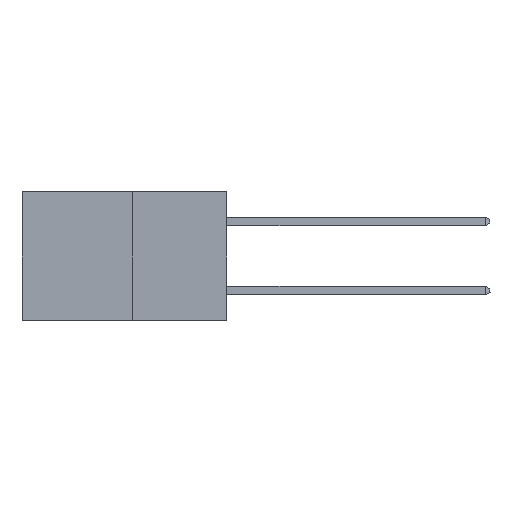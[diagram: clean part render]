
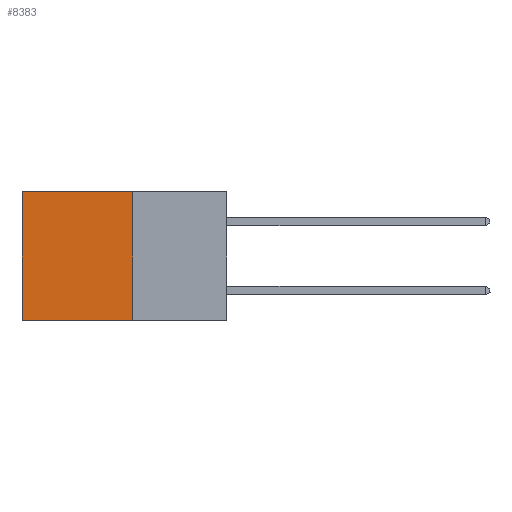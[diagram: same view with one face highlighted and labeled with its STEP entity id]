
A CAD part, left-side view. The second image highlights one B-rep face of the part: STEP entity #8383.
In plain terms, the highlighted planar face has unit normal (-1, 0, 0).
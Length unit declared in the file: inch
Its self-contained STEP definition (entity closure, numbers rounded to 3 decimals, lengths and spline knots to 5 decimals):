
#477 = ORIENTED_EDGE ( 'NONE', *, *, #12826, .F. ) ;
#1267 = VECTOR ( 'NONE', #27834, 39.37008 ) ;
#1766 = DIRECTION ( 'NONE',  ( 0., 0., -1. ) ) ;
#3061 = EDGE_CURVE ( 'NONE', #23658, #22537, #20502, .T. ) ;
#3997 = CARTESIAN_POINT ( 'NONE',  ( 0.277, 0.59, -0.37 ) ) ;
#6539 = LINE ( 'NONE', #20840, #18861 ) ;
#6622 = DIRECTION ( 'NONE',  ( 0., 0., -1. ) ) ;
#6968 = DIRECTION ( 'NONE',  ( 0., 0., -1. ) ) ;
#8383 = ADVANCED_FACE ( 'NONE', ( #29174 ), #13370, .F. ) ;
#8537 = EDGE_CURVE ( 'NONE', #22537, #20049, #6539, .T. ) ;
#9358 = CARTESIAN_POINT ( 'NONE',  ( 0.277, 0.27, -0.37 ) ) ;
#9962 = CARTESIAN_POINT ( 'NONE',  ( 0.277, 0.27, 0. ) ) ;
#10713 = ORIENTED_EDGE ( 'NONE', *, *, #3061, .T. ) ;
#11480 = DIRECTION ( 'NONE',  ( 0., 1., 0. ) ) ;
#12826 = EDGE_CURVE ( 'NONE', #23658, #17734, #27146, .T. ) ;
#13370 = PLANE ( 'NONE',  #28268 ) ;
#14261 = VECTOR ( 'NONE', #6622, 39.37008 ) ;
#15702 = DIRECTION ( 'NONE',  ( 1., 0., 0. ) ) ;
#16728 = CARTESIAN_POINT ( 'NONE',  ( 0.277, 0.59, 0. ) ) ;
#17734 = VERTEX_POINT ( 'NONE', #9358 ) ;
#17943 = ORIENTED_EDGE ( 'NONE', *, *, #8537, .T. ) ;
#18240 = EDGE_LOOP ( 'NONE', ( #17943, #22603, #477, #10713 ) ) ;
#18861 = VECTOR ( 'NONE', #6968, 39.37008 ) ;
#20049 = VERTEX_POINT ( 'NONE', #3997 ) ;
#20240 = CARTESIAN_POINT ( 'NONE',  ( 0.277, 0.27, -0.37 ) ) ;
#20502 = LINE ( 'NONE', #9962, #1267 ) ;
#20840 = CARTESIAN_POINT ( 'NONE',  ( 0.277, 0.59, -0.37 ) ) ;
#22537 = VERTEX_POINT ( 'NONE', #16728 ) ;
#22603 = ORIENTED_EDGE ( 'NONE', *, *, #29498, .F. ) ;
#23658 = VERTEX_POINT ( 'NONE', #27513 ) ;
#25047 = CARTESIAN_POINT ( 'NONE',  ( 0.277, 0.27, -0.37 ) ) ;
#25210 = CARTESIAN_POINT ( 'NONE',  ( 0.277, 0.27, -0.37 ) ) ;
#26482 = VECTOR ( 'NONE', #11480, 39.37008 ) ;
#27146 = LINE ( 'NONE', #25047, #14261 ) ;
#27167 = LINE ( 'NONE', #25210, #26482 ) ;
#27513 = CARTESIAN_POINT ( 'NONE',  ( 0.277, 0.27, 0. ) ) ;
#27834 = DIRECTION ( 'NONE',  ( 0., 1., 0. ) ) ;
#28268 = AXIS2_PLACEMENT_3D ( 'NONE', #20240, #15702, #1766 ) ;
#29174 = FACE_OUTER_BOUND ( 'NONE', #18240, .T. ) ;
#29498 = EDGE_CURVE ( 'NONE', #17734, #20049, #27167, .T. ) ;
